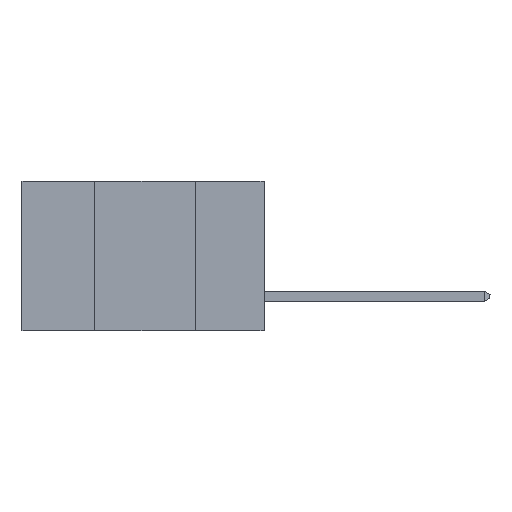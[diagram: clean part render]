
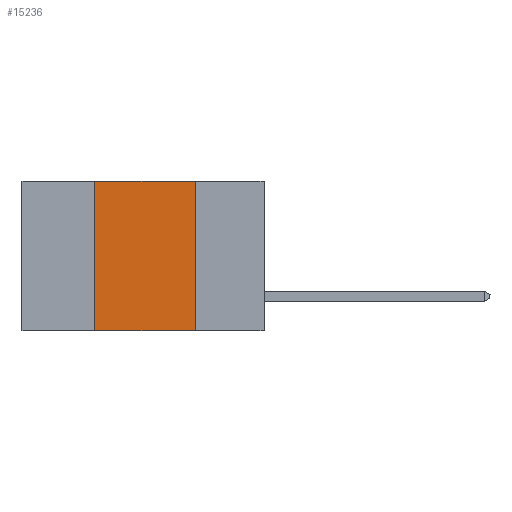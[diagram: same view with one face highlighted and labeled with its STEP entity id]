
A CAD part, left-side view. The second image highlights one B-rep face of the part: STEP entity #15236.
In plain terms, the highlighted planar face has unit normal (-1, 0, 0).
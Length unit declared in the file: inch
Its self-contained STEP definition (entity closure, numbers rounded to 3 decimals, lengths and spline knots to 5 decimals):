
#90 = EDGE_CURVE ( 'NONE', #2042, #1449, #10259, .T. ) ;
#739 = CARTESIAN_POINT ( 'NONE',  ( 0., 0.17, -0.37 ) ) ;
#828 = ORIENTED_EDGE ( 'NONE', *, *, #6739, .F. ) ;
#1175 = DIRECTION ( 'NONE',  ( 0., -1., 0. ) ) ;
#1176 = CARTESIAN_POINT ( 'NONE',  ( 0., 0.42, 0. ) ) ;
#1219 = ORIENTED_EDGE ( 'NONE', *, *, #90, .T. ) ;
#1449 = VERTEX_POINT ( 'NONE', #739 ) ;
#2042 = VERTEX_POINT ( 'NONE', #7609 ) ;
#2411 = CARTESIAN_POINT ( 'NONE',  ( 0., 0.17, -0.37 ) ) ;
#3215 = DIRECTION ( 'NONE',  ( 0., 0., 1. ) ) ;
#3271 = LINE ( 'NONE', #10721, #7003 ) ;
#3701 = AXIS2_PLACEMENT_3D ( 'NONE', #10467, #14304, #13112 ) ;
#4178 = CARTESIAN_POINT ( 'NONE',  ( 0., 0.6, -0.37 ) ) ;
#4316 = PLANE ( 'NONE',  #3701 ) ;
#4352 = LINE ( 'NONE', #14181, #5162 ) ;
#5162 = VECTOR ( 'NONE', #3215, 39.37008 ) ;
#5863 = FACE_OUTER_BOUND ( 'NONE', #13076, .T. ) ;
#6329 = VECTOR ( 'NONE', #7374, 39.37008 ) ;
#6739 = EDGE_CURVE ( 'NONE', #2042, #8575, #4352, .T. ) ;
#7003 = VECTOR ( 'NONE', #1175, 39.37008 ) ;
#7199 = EDGE_CURVE ( 'NONE', #8575, #14194, #3271, .T. ) ;
#7374 = DIRECTION ( 'NONE',  ( 0., 0., -1. ) ) ;
#7609 = CARTESIAN_POINT ( 'NONE',  ( 0., 0.42, -0.37 ) ) ;
#8575 = VERTEX_POINT ( 'NONE', #1176 ) ;
#9327 = ORIENTED_EDGE ( 'NONE', *, *, #15825, .F. ) ;
#9933 = LINE ( 'NONE', #2411, #6329 ) ;
#10259 = LINE ( 'NONE', #4178, #11232 ) ;
#10467 = CARTESIAN_POINT ( 'NONE',  ( 0., 0.6, 0. ) ) ;
#10721 = CARTESIAN_POINT ( 'NONE',  ( 0., 0.6, 0. ) ) ;
#11232 = VECTOR ( 'NONE', #13778, 39.37008 ) ;
#12634 = ORIENTED_EDGE ( 'NONE', *, *, #7199, .F. ) ;
#13076 = EDGE_LOOP ( 'NONE', ( #9327, #12634, #828, #1219 ) ) ;
#13112 = DIRECTION ( 'NONE',  ( 0., 0., -1. ) ) ;
#13778 = DIRECTION ( 'NONE',  ( 0., -1., 0. ) ) ;
#14181 = CARTESIAN_POINT ( 'NONE',  ( 0., 0.42, -0.37 ) ) ;
#14194 = VERTEX_POINT ( 'NONE', #15076 ) ;
#14304 = DIRECTION ( 'NONE',  ( 1., 0., 0. ) ) ;
#15076 = CARTESIAN_POINT ( 'NONE',  ( 0., 0.17, 0. ) ) ;
#15236 = ADVANCED_FACE ( 'NONE', ( #5863 ), #4316, .F. ) ;
#15825 = EDGE_CURVE ( 'NONE', #14194, #1449, #9933, .T. ) ;
